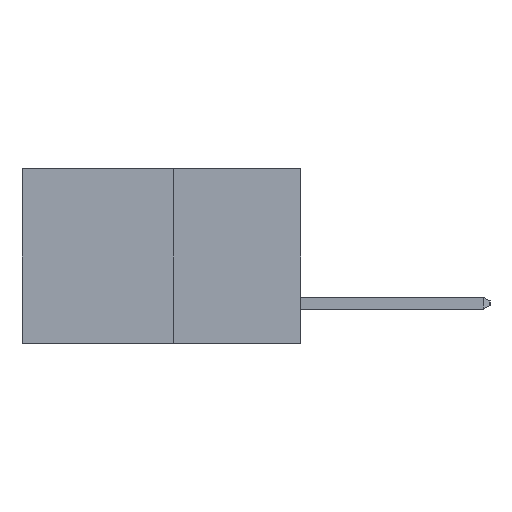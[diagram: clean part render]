
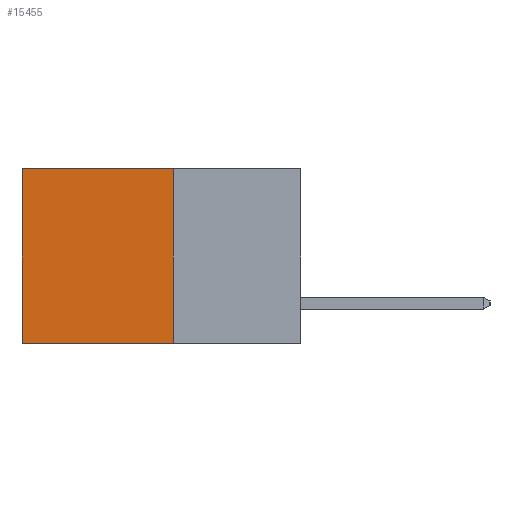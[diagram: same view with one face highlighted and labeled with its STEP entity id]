
A CAD part, left-side view. The second image highlights one B-rep face of the part: STEP entity #15455.
In plain terms, the highlighted planar face has unit normal (-1, 0, 0).
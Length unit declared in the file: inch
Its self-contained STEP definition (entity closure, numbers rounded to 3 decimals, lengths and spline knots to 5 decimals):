
#1076 = EDGE_CURVE ( 'NONE', #19500, #5546, #19791, .T. ) ;
#1149 = CARTESIAN_POINT ( 'NONE',  ( 0.277, 0.27, -0.37 ) ) ;
#1413 = ORIENTED_EDGE ( 'NONE', *, *, #11191, .F. ) ;
#2498 = VERTEX_POINT ( 'NONE', #15473 ) ;
#2833 = DIRECTION ( 'NONE',  ( 0., 1., 0. ) ) ;
#3689 = EDGE_CURVE ( 'NONE', #18495, #19500, #20176, .T. ) ;
#4484 = DIRECTION ( 'NONE',  ( 0., 0., -1. ) ) ;
#4555 = PLANE ( 'NONE',  #10775 ) ;
#5154 = FACE_OUTER_BOUND ( 'NONE', #20868, .T. ) ;
#5546 = VERTEX_POINT ( 'NONE', #11987 ) ;
#6015 = CARTESIAN_POINT ( 'NONE',  ( 0.277, 0.27, 0. ) ) ;
#6881 = CARTESIAN_POINT ( 'NONE',  ( 0.277, 0.59, 0. ) ) ;
#7695 = ORIENTED_EDGE ( 'NONE', *, *, #15408, .F. ) ;
#8075 = DIRECTION ( 'NONE',  ( 0., 1., 0. ) ) ;
#9452 = CARTESIAN_POINT ( 'NONE',  ( 0.277, 0.27, -0.37 ) ) ;
#10199 = ORIENTED_EDGE ( 'NONE', *, *, #3689, .T. ) ;
#10775 = AXIS2_PLACEMENT_3D ( 'NONE', #9452, #20887, #11112 ) ;
#11014 = VECTOR ( 'NONE', #4484, 39.37008 ) ;
#11112 = DIRECTION ( 'NONE',  ( 0., 0., -1. ) ) ;
#11122 = ORIENTED_EDGE ( 'NONE', *, *, #1076, .T. ) ;
#11191 = EDGE_CURVE ( 'NONE', #2498, #5546, #14230, .T. ) ;
#11987 = CARTESIAN_POINT ( 'NONE',  ( 0.277, 0.59, -0.37 ) ) ;
#13964 = CARTESIAN_POINT ( 'NONE',  ( 0.277, 0.27, 0. ) ) ;
#14230 = LINE ( 'NONE', #14298, #18565 ) ;
#14298 = CARTESIAN_POINT ( 'NONE',  ( 0.277, 0.27, -0.37 ) ) ;
#15408 = EDGE_CURVE ( 'NONE', #18495, #2498, #19198, .T. ) ;
#15455 = ADVANCED_FACE ( 'NONE', ( #5154 ), #4555, .F. ) ;
#15473 = CARTESIAN_POINT ( 'NONE',  ( 0.277, 0.27, -0.37 ) ) ;
#15498 = VECTOR ( 'NONE', #18079, 39.37008 ) ;
#16389 = VECTOR ( 'NONE', #8075, 39.37008 ) ;
#18079 = DIRECTION ( 'NONE',  ( 0., 0., -1. ) ) ;
#18495 = VERTEX_POINT ( 'NONE', #6015 ) ;
#18565 = VECTOR ( 'NONE', #2833, 39.37008 ) ;
#19198 = LINE ( 'NONE', #1149, #11014 ) ;
#19500 = VERTEX_POINT ( 'NONE', #6881 ) ;
#19549 = CARTESIAN_POINT ( 'NONE',  ( 0.277, 0.59, -0.37 ) ) ;
#19791 = LINE ( 'NONE', #19549, #15498 ) ;
#20176 = LINE ( 'NONE', #13964, #16389 ) ;
#20868 = EDGE_LOOP ( 'NONE', ( #11122, #1413, #7695, #10199 ) ) ;
#20887 = DIRECTION ( 'NONE',  ( 1., 0., 0. ) ) ;
